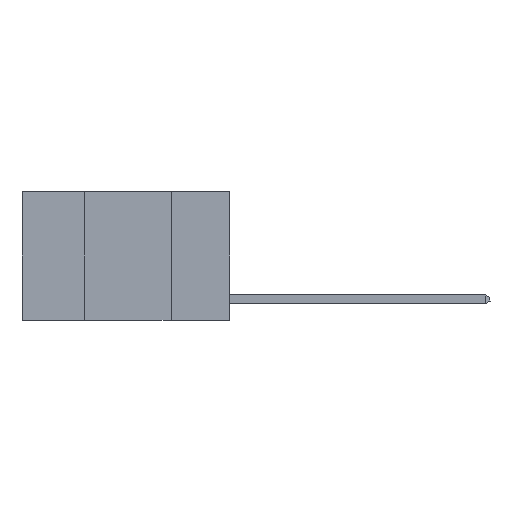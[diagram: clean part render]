
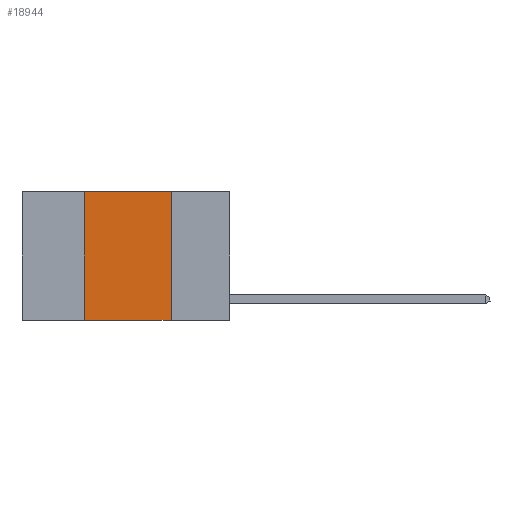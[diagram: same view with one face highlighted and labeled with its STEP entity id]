
A CAD part, left-side view. The second image highlights one B-rep face of the part: STEP entity #18944.
In plain terms, the highlighted planar face has unit normal (-1, 0, 0).
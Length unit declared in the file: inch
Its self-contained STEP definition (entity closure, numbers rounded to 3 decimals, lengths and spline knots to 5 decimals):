
#226 = LINE ( 'NONE', #11014, #19494 ) ;
#954 = CARTESIAN_POINT ( 'NONE',  ( 0., 0.6, 0. ) ) ;
#1333 = CARTESIAN_POINT ( 'NONE',  ( 0., 0.17, 0. ) ) ;
#2058 = DIRECTION ( 'NONE',  ( 0., 0., 1. ) ) ;
#4062 = ORIENTED_EDGE ( 'NONE', *, *, #15584, .F. ) ;
#4750 = CARTESIAN_POINT ( 'NONE',  ( 0., 0.6, -0.37 ) ) ;
#5707 = LINE ( 'NONE', #954, #13506 ) ;
#5814 = DIRECTION ( 'NONE',  ( 0., -1., 0. ) ) ;
#6397 = EDGE_CURVE ( 'NONE', #8827, #7795, #18411, .T. ) ;
#7252 = CARTESIAN_POINT ( 'NONE',  ( 0., 0.6, 0. ) ) ;
#7795 = VERTEX_POINT ( 'NONE', #15200 ) ;
#8055 = CARTESIAN_POINT ( 'NONE',  ( 0., 0.42, -0.37 ) ) ;
#8484 = ORIENTED_EDGE ( 'NONE', *, *, #15020, .T. ) ;
#8827 = VERTEX_POINT ( 'NONE', #8055 ) ;
#8869 = PLANE ( 'NONE',  #12494 ) ;
#8924 = VERTEX_POINT ( 'NONE', #1333 ) ;
#9376 = LINE ( 'NONE', #4750, #10137 ) ;
#10137 = VECTOR ( 'NONE', #13862, 39.37008 ) ;
#10264 = EDGE_CURVE ( 'NONE', #7795, #8924, #5707, .T. ) ;
#10539 = DIRECTION ( 'NONE',  ( 1., 0., 0. ) ) ;
#11014 = CARTESIAN_POINT ( 'NONE',  ( 0., 0.17, 0. ) ) ;
#11544 = ORIENTED_EDGE ( 'NONE', *, *, #6397, .F. ) ;
#11639 = VECTOR ( 'NONE', #2058, 39.37008 ) ;
#11696 = ORIENTED_EDGE ( 'NONE', *, *, #10264, .F. ) ;
#12494 = AXIS2_PLACEMENT_3D ( 'NONE', #7252, #10539, #13342 ) ;
#13342 = DIRECTION ( 'NONE',  ( 0., 0., -1. ) ) ;
#13506 = VECTOR ( 'NONE', #5814, 39.37008 ) ;
#13862 = DIRECTION ( 'NONE',  ( 0., -1., 0. ) ) ;
#13998 = VERTEX_POINT ( 'NONE', #19406 ) ;
#14055 = CARTESIAN_POINT ( 'NONE',  ( 0., 0.42, 0. ) ) ;
#14096 = EDGE_LOOP ( 'NONE', ( #4062, #11696, #11544, #8484 ) ) ;
#15020 = EDGE_CURVE ( 'NONE', #8827, #13998, #9376, .T. ) ;
#15200 = CARTESIAN_POINT ( 'NONE',  ( 0., 0.42, 0. ) ) ;
#15584 = EDGE_CURVE ( 'NONE', #8924, #13998, #226, .T. ) ;
#16389 = FACE_OUTER_BOUND ( 'NONE', #14096, .T. ) ;
#17036 = DIRECTION ( 'NONE',  ( 0., 0., -1. ) ) ;
#18411 = LINE ( 'NONE', #14055, #11639 ) ;
#18944 = ADVANCED_FACE ( 'NONE', ( #16389 ), #8869, .F. ) ;
#19406 = CARTESIAN_POINT ( 'NONE',  ( 0., 0.17, -0.37 ) ) ;
#19494 = VECTOR ( 'NONE', #17036, 39.37008 ) ;
